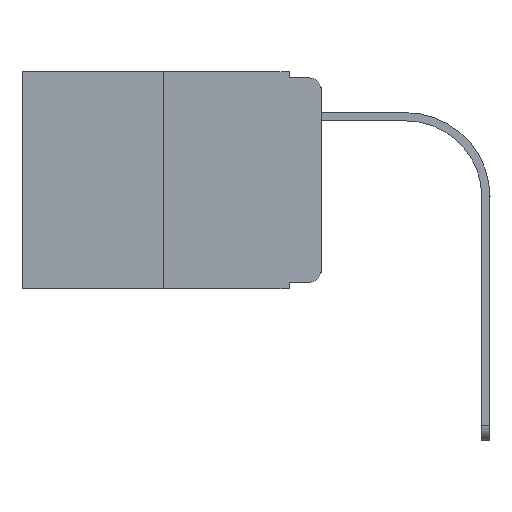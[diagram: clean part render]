
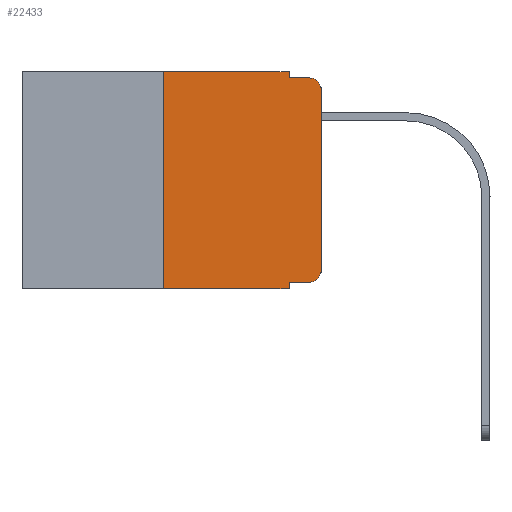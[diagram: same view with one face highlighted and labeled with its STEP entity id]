
A CAD part, left-side view. The second image highlights one B-rep face of the part: STEP entity #22433.
In plain terms, the highlighted planar face has unit normal (-1, 0, 0).
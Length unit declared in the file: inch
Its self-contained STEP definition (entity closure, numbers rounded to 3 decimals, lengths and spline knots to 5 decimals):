
#581 = CARTESIAN_POINT ( 'NONE',  ( 0., 0.051, -0.333 ) ) ;
#587 = LINE ( 'NONE', #16768, #16863 ) ;
#637 = VECTOR ( 'NONE', #3679, 39.37008 ) ;
#676 = FACE_OUTER_BOUND ( 'NONE', #22556, .T. ) ;
#743 = CARTESIAN_POINT ( 'NONE',  ( 0., 0.051, -0.01 ) ) ;
#784 = ORIENTED_EDGE ( 'NONE', *, *, #6472, .F. ) ;
#800 = DIRECTION ( 'NONE',  ( 0., 0., -1. ) ) ;
#947 = VERTEX_POINT ( 'NONE', #581 ) ;
#987 = VECTOR ( 'NONE', #23948, 39.37008 ) ;
#1187 = DIRECTION ( 'NONE',  ( 0., 0., -1. ) ) ;
#1462 = LINE ( 'NONE', #18945, #10454 ) ;
#2073 = LINE ( 'NONE', #15542, #18600 ) ;
#2720 = EDGE_CURVE ( 'NONE', #947, #7484, #1462, .T. ) ;
#3679 = DIRECTION ( 'NONE',  ( 0., -1., 0. ) ) ;
#4147 = DIRECTION ( 'NONE',  ( 0., 0., 1. ) ) ;
#4739 = VECTOR ( 'NONE', #25303, 39.37008 ) ;
#5171 = ORIENTED_EDGE ( 'NONE', *, *, #21007, .T. ) ;
#5680 = LINE ( 'NONE', #17718, #20860 ) ;
#6208 = CARTESIAN_POINT ( 'NONE',  ( 0., 0.02, -0.03 ) ) ;
#6472 = EDGE_CURVE ( 'NONE', #9830, #19248, #18550, .T. ) ;
#6509 = AXIS2_PLACEMENT_3D ( 'NONE', #6208, #14107, #10342 ) ;
#6760 = ORIENTED_EDGE ( 'NONE', *, *, #11522, .T. ) ;
#7334 = CIRCLE ( 'NONE', #6509, 0.02 ) ;
#7428 = DIRECTION ( 'NONE',  ( 0., 0., -1. ) ) ;
#7484 = VERTEX_POINT ( 'NONE', #14852 ) ;
#8280 = EDGE_CURVE ( 'NONE', #20899, #18559, #2073, .T. ) ;
#8700 = DIRECTION ( 'NONE',  ( 0., 0., -1. ) ) ;
#8958 = DIRECTION ( 'NONE',  ( -1., 0., 0. ) ) ;
#9015 = DIRECTION ( 'NONE',  ( 0., 0., 1. ) ) ;
#9166 = CARTESIAN_POINT ( 'NONE',  ( 0., 0.051, 0. ) ) ;
#9708 = VECTOR ( 'NONE', #8700, 39.37008 ) ;
#9830 = VERTEX_POINT ( 'NONE', #9166 ) ;
#10253 = CARTESIAN_POINT ( 'NONE',  ( 0., 0.02, -0.01 ) ) ;
#10342 = DIRECTION ( 'NONE',  ( 0., 0., -1. ) ) ;
#10454 = VECTOR ( 'NONE', #7428, 39.37008 ) ;
#10647 = CARTESIAN_POINT ( 'NONE',  ( 0., 0.02, -0.313 ) ) ;
#10742 = ORIENTED_EDGE ( 'NONE', *, *, #17702, .F. ) ;
#11212 = CARTESIAN_POINT ( 'NONE',  ( 0., 0.051, -0.333 ) ) ;
#11363 = CARTESIAN_POINT ( 'NONE',  ( 0., 0.02, -0.333 ) ) ;
#11522 = EDGE_CURVE ( 'NONE', #947, #21397, #18986, .T. ) ;
#11645 = CARTESIAN_POINT ( 'NONE',  ( 0., 0., -0.313 ) ) ;
#12465 = ORIENTED_EDGE ( 'NONE', *, *, #2720, .F. ) ;
#13324 = ORIENTED_EDGE ( 'NONE', *, *, #8280, .T. ) ;
#13579 = DIRECTION ( 'NONE',  ( 0., -1., 0. ) ) ;
#13946 = ORIENTED_EDGE ( 'NONE', *, *, #23723, .T. ) ;
#13994 = LINE ( 'NONE', #23825, #987 ) ;
#14107 = DIRECTION ( 'NONE',  ( -1., 0., 0. ) ) ;
#14637 = CARTESIAN_POINT ( 'NONE',  ( 0., 0.051, 0. ) ) ;
#14852 = CARTESIAN_POINT ( 'NONE',  ( 0., 0.051, -0.343 ) ) ;
#15542 = CARTESIAN_POINT ( 'NONE',  ( 0., 0., 0. ) ) ;
#15722 = EDGE_CURVE ( 'NONE', #20774, #25418, #587, .T. ) ;
#16007 = VERTEX_POINT ( 'NONE', #10253 ) ;
#16726 = LINE ( 'NONE', #22705, #637 ) ;
#16768 = CARTESIAN_POINT ( 'NONE',  ( 0., 0.25, 0. ) ) ;
#16852 = DIRECTION ( 'NONE',  ( 1., 0., 0. ) ) ;
#16863 = VECTOR ( 'NONE', #9015, 39.37008 ) ;
#17702 = EDGE_CURVE ( 'NONE', #25418, #9830, #5680, .T. ) ;
#17718 = CARTESIAN_POINT ( 'NONE',  ( 0., 0.473, 0. ) ) ;
#18550 = LINE ( 'NONE', #14637, #9708 ) ;
#18559 = VERTEX_POINT ( 'NONE', #21779 ) ;
#18600 = VECTOR ( 'NONE', #4147, 39.37008 ) ;
#18945 = CARTESIAN_POINT ( 'NONE',  ( 0., 0.051, 0. ) ) ;
#18986 = LINE ( 'NONE', #11212, #4739 ) ;
#19248 = VERTEX_POINT ( 'NONE', #743 ) ;
#19752 = EDGE_CURVE ( 'NONE', #19248, #16007, #16726, .T. ) ;
#20415 = AXIS2_PLACEMENT_3D ( 'NONE', #10647, #8958, #1187 ) ;
#20595 = CARTESIAN_POINT ( 'NONE',  ( 0., 0.473, 0. ) ) ;
#20774 = VERTEX_POINT ( 'NONE', #20871 ) ;
#20860 = VECTOR ( 'NONE', #13579, 39.37008 ) ;
#20871 = CARTESIAN_POINT ( 'NONE',  ( 0., 0.25, -0.343 ) ) ;
#20899 = VERTEX_POINT ( 'NONE', #11645 ) ;
#20973 = ORIENTED_EDGE ( 'NONE', *, *, #15722, .F. ) ;
#21007 = EDGE_CURVE ( 'NONE', #18559, #16007, #7334, .T. ) ;
#21397 = VERTEX_POINT ( 'NONE', #11363 ) ;
#21779 = CARTESIAN_POINT ( 'NONE',  ( 0., 0., -0.03 ) ) ;
#21861 = ORIENTED_EDGE ( 'NONE', *, *, #25125, .T. ) ;
#22433 = ADVANCED_FACE ( 'NONE', ( #676 ), #22543, .F. ) ;
#22435 = ORIENTED_EDGE ( 'NONE', *, *, #19752, .F. ) ;
#22543 = PLANE ( 'NONE',  #24499 ) ;
#22556 = EDGE_LOOP ( 'NONE', ( #13324, #5171, #22435, #784, #10742, #20973, #21861, #12465, #6760, #13946 ) ) ;
#22705 = CARTESIAN_POINT ( 'NONE',  ( 0., 0.051, -0.01 ) ) ;
#23634 = CARTESIAN_POINT ( 'NONE',  ( 0., 0.25, 0. ) ) ;
#23723 = EDGE_CURVE ( 'NONE', #21397, #20899, #24557, .T. ) ;
#23825 = CARTESIAN_POINT ( 'NONE',  ( 0., 0.473, -0.343 ) ) ;
#23948 = DIRECTION ( 'NONE',  ( 0., -1., 0. ) ) ;
#24499 = AXIS2_PLACEMENT_3D ( 'NONE', #20595, #16852, #800 ) ;
#24557 = CIRCLE ( 'NONE', #20415, 0.02 ) ;
#25125 = EDGE_CURVE ( 'NONE', #20774, #7484, #13994, .T. ) ;
#25303 = DIRECTION ( 'NONE',  ( 0., -1., 0. ) ) ;
#25418 = VERTEX_POINT ( 'NONE', #23634 ) ;
